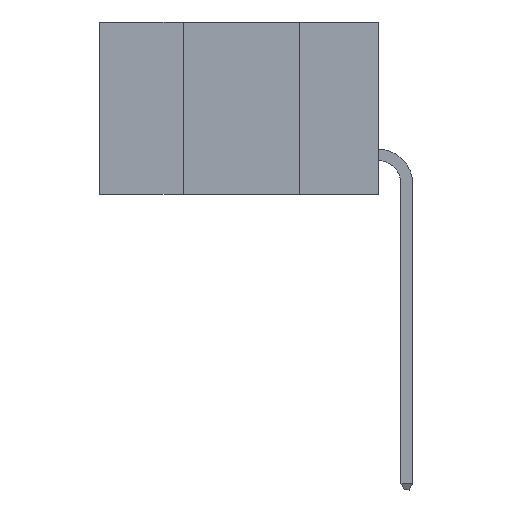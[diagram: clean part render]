
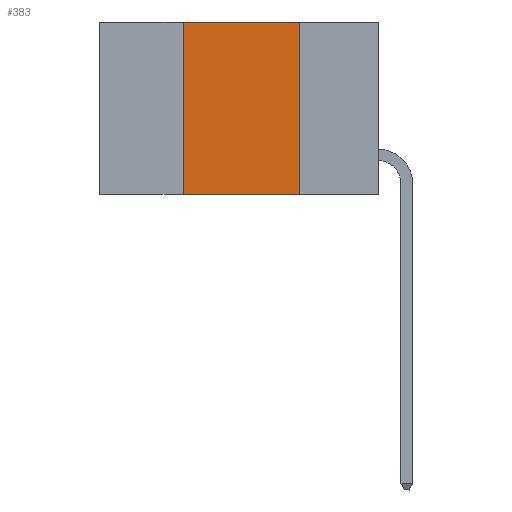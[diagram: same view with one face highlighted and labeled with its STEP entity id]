
A CAD part, left-side view. The second image highlights one B-rep face of the part: STEP entity #383.
In plain terms, the highlighted planar face has unit normal (-1, 0, 0).
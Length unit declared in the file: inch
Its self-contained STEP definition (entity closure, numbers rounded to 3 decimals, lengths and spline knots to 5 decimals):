
#126 = DIRECTION ( 'NONE',  ( 0., -1., 0. ) ) ;
#367 = VERTEX_POINT ( 'NONE', #3359 ) ;
#383 = ADVANCED_FACE ( 'NONE', ( #5279 ), #4430, .F. ) ;
#947 = DIRECTION ( 'NONE',  ( 0., 0., 1. ) ) ;
#1021 = EDGE_CURVE ( 'NONE', #9061, #8054, #3683, .T. ) ;
#1157 = CARTESIAN_POINT ( 'NONE',  ( 0., 0.17, 0. ) ) ;
#1389 = ORIENTED_EDGE ( 'NONE', *, *, #1021, .T. ) ;
#1845 = ORIENTED_EDGE ( 'NONE', *, *, #9468, .F. ) ;
#1953 = CARTESIAN_POINT ( 'NONE',  ( 0., 0.17, 0. ) ) ;
#2178 = DIRECTION ( 'NONE',  ( 0., 0., -1. ) ) ;
#2642 = CARTESIAN_POINT ( 'NONE',  ( 0., 0.6, 0. ) ) ;
#2977 = EDGE_CURVE ( 'NONE', #3016, #8054, #11884, .T. ) ;
#3016 = VERTEX_POINT ( 'NONE', #1953 ) ;
#3066 = DIRECTION ( 'NONE',  ( 0., 0., -1. ) ) ;
#3084 = DIRECTION ( 'NONE',  ( 1., 0., 0. ) ) ;
#3359 = CARTESIAN_POINT ( 'NONE',  ( 0., 0.42, 0. ) ) ;
#3683 = LINE ( 'NONE', #9227, #10683 ) ;
#4230 = EDGE_LOOP ( 'NONE', ( #8273, #10719, #1845, #1389 ) ) ;
#4430 = PLANE ( 'NONE',  #6624 ) ;
#4726 = EDGE_CURVE ( 'NONE', #367, #3016, #7434, .T. ) ;
#5279 = FACE_OUTER_BOUND ( 'NONE', #4230, .T. ) ;
#6624 = AXIS2_PLACEMENT_3D ( 'NONE', #2642, #3084, #3066 ) ;
#6952 = VECTOR ( 'NONE', #2178, 39.37008 ) ;
#7040 = VECTOR ( 'NONE', #947, 39.37008 ) ;
#7434 = LINE ( 'NONE', #9795, #9451 ) ;
#8054 = VERTEX_POINT ( 'NONE', #8088 ) ;
#8088 = CARTESIAN_POINT ( 'NONE',  ( 0., 0.17, -0.37 ) ) ;
#8273 = ORIENTED_EDGE ( 'NONE', *, *, #2977, .F. ) ;
#9061 = VERTEX_POINT ( 'NONE', #10860 ) ;
#9227 = CARTESIAN_POINT ( 'NONE',  ( 0., 0.6, -0.37 ) ) ;
#9451 = VECTOR ( 'NONE', #11717, 39.37008 ) ;
#9468 = EDGE_CURVE ( 'NONE', #9061, #367, #12265, .T. ) ;
#9795 = CARTESIAN_POINT ( 'NONE',  ( 0., 0.6, 0. ) ) ;
#10576 = CARTESIAN_POINT ( 'NONE',  ( 0., 0.42, 0. ) ) ;
#10683 = VECTOR ( 'NONE', #126, 39.37008 ) ;
#10719 = ORIENTED_EDGE ( 'NONE', *, *, #4726, .F. ) ;
#10860 = CARTESIAN_POINT ( 'NONE',  ( 0., 0.42, -0.37 ) ) ;
#11717 = DIRECTION ( 'NONE',  ( 0., -1., 0. ) ) ;
#11884 = LINE ( 'NONE', #1157, #6952 ) ;
#12265 = LINE ( 'NONE', #10576, #7040 ) ;
